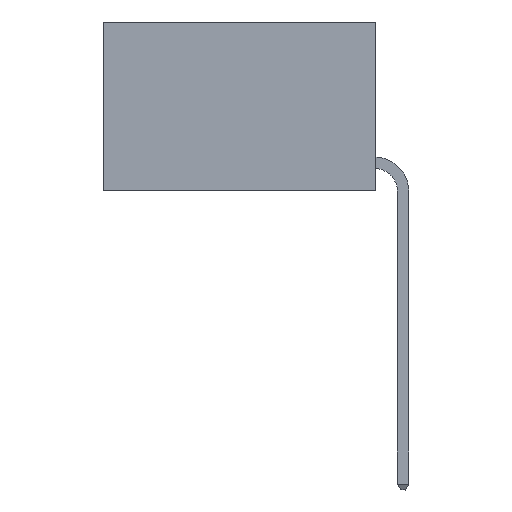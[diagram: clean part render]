
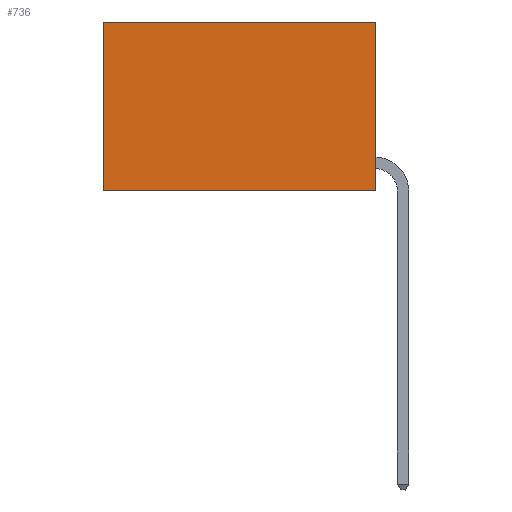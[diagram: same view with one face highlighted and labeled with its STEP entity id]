
A CAD part, left-side view. The second image highlights one B-rep face of the part: STEP entity #736.
In plain terms, the highlighted planar face has unit normal (-1, 0, 0).
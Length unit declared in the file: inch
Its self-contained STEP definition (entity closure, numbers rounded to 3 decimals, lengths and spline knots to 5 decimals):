
#7 = LINE ( 'NONE', #4194, #3377 ) ;
#311 = VECTOR ( 'NONE', #4922, 39.37008 ) ;
#595 = CARTESIAN_POINT ( 'NONE',  ( 0.2625, 0., -0.37 ) ) ;
#610 = LINE ( 'NONE', #10690, #4822 ) ;
#736 = ADVANCED_FACE ( 'NONE', ( #16141 ), #3315, .F. ) ;
#1619 = EDGE_CURVE ( 'NONE', #16520, #4377, #11370, .T. ) ;
#3315 = PLANE ( 'NONE',  #13731 ) ;
#3377 = VECTOR ( 'NONE', #6913, 39.37008 ) ;
#3397 = VERTEX_POINT ( 'NONE', #3840 ) ;
#3840 = CARTESIAN_POINT ( 'NONE',  ( 0.2625, 0.6, 0. ) ) ;
#3852 = DIRECTION ( 'NONE',  ( 0., 1., 0. ) ) ;
#4122 = EDGE_CURVE ( 'NONE', #17549, #16520, #7, .T. ) ;
#4194 = CARTESIAN_POINT ( 'NONE',  ( 0.2625, 0., 0. ) ) ;
#4377 = VERTEX_POINT ( 'NONE', #11582 ) ;
#4545 = LINE ( 'NONE', #12677, #14855 ) ;
#4822 = VECTOR ( 'NONE', #3852, 39.37008 ) ;
#4922 = DIRECTION ( 'NONE',  ( 0., 1., 0. ) ) ;
#6704 = DIRECTION ( 'NONE',  ( 1., 0., 0. ) ) ;
#6913 = DIRECTION ( 'NONE',  ( 0., 0., -1. ) ) ;
#6959 = CARTESIAN_POINT ( 'NONE',  ( 0.2625, 0., 0. ) ) ;
#9775 = ORIENTED_EDGE ( 'NONE', *, *, #4122, .F. ) ;
#10690 = CARTESIAN_POINT ( 'NONE',  ( 0.2625, 0., 0. ) ) ;
#11370 = LINE ( 'NONE', #595, #311 ) ;
#11519 = CARTESIAN_POINT ( 'NONE',  ( 0.2625, 0., -0.37 ) ) ;
#11582 = CARTESIAN_POINT ( 'NONE',  ( 0.2625, 0.6, -0.37 ) ) ;
#11645 = EDGE_CURVE ( 'NONE', #3397, #4377, #4545, .T. ) ;
#12097 = ORIENTED_EDGE ( 'NONE', *, *, #11645, .T. ) ;
#12677 = CARTESIAN_POINT ( 'NONE',  ( 0.2625, 0.6, 0. ) ) ;
#13342 = EDGE_LOOP ( 'NONE', ( #12097, #16121, #9775, #13385 ) ) ;
#13385 = ORIENTED_EDGE ( 'NONE', *, *, #16765, .T. ) ;
#13731 = AXIS2_PLACEMENT_3D ( 'NONE', #6959, #6704, #15195 ) ;
#14010 = DIRECTION ( 'NONE',  ( 0., 0., -1. ) ) ;
#14855 = VECTOR ( 'NONE', #14010, 39.37008 ) ;
#15195 = DIRECTION ( 'NONE',  ( 0., 0., -1. ) ) ;
#16107 = CARTESIAN_POINT ( 'NONE',  ( 0.2625, 0., 0. ) ) ;
#16121 = ORIENTED_EDGE ( 'NONE', *, *, #1619, .F. ) ;
#16141 = FACE_OUTER_BOUND ( 'NONE', #13342, .T. ) ;
#16520 = VERTEX_POINT ( 'NONE', #11519 ) ;
#16765 = EDGE_CURVE ( 'NONE', #17549, #3397, #610, .T. ) ;
#17549 = VERTEX_POINT ( 'NONE', #16107 ) ;
